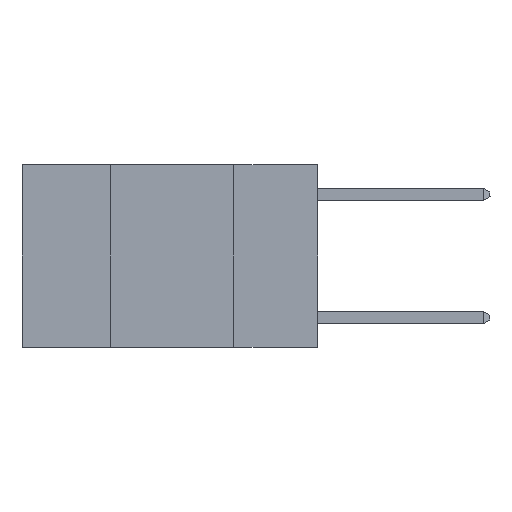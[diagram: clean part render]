
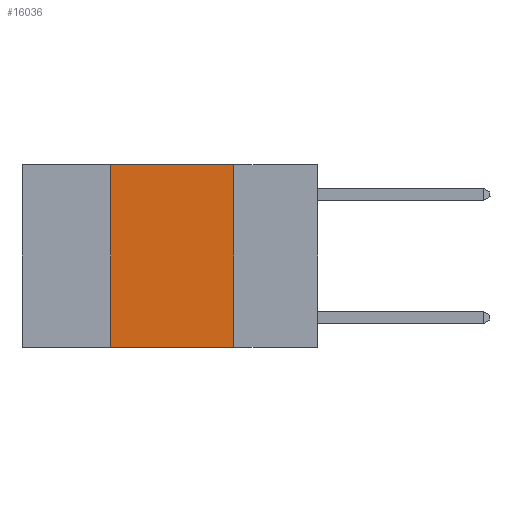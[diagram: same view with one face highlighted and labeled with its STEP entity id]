
A CAD part, left-side view. The second image highlights one B-rep face of the part: STEP entity #16036.
In plain terms, the highlighted planar face has unit normal (-1, 0, 0).
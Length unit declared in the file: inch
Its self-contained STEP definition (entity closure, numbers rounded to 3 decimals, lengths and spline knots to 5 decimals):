
#770 = CARTESIAN_POINT ( 'NONE',  ( 0., 0.42, 0. ) ) ;
#827 = VECTOR ( 'NONE', #1540, 39.37008 ) ;
#918 = LINE ( 'NONE', #11478, #5633 ) ;
#1540 = DIRECTION ( 'NONE',  ( 0., -1., 0. ) ) ;
#2212 = DIRECTION ( 'NONE',  ( 1., 0., 0. ) ) ;
#2724 = CARTESIAN_POINT ( 'NONE',  ( 0., 0.17, -0.37 ) ) ;
#3726 = EDGE_CURVE ( 'NONE', #4043, #10433, #17249, .T. ) ;
#4043 = VERTEX_POINT ( 'NONE', #13891 ) ;
#4356 = DIRECTION ( 'NONE',  ( 0., 0., -1. ) ) ;
#4636 = VECTOR ( 'NONE', #4356, 39.37008 ) ;
#5186 = AXIS2_PLACEMENT_3D ( 'NONE', #9815, #2212, #9720 ) ;
#5633 = VECTOR ( 'NONE', #13064, 39.37008 ) ;
#5973 = CARTESIAN_POINT ( 'NONE',  ( 0., 0.42, 0. ) ) ;
#7936 = FACE_OUTER_BOUND ( 'NONE', #10590, .T. ) ;
#8312 = CARTESIAN_POINT ( 'NONE',  ( 0., 0.17, 0. ) ) ;
#8603 = VERTEX_POINT ( 'NONE', #2724 ) ;
#8655 = EDGE_CURVE ( 'NONE', #10433, #9230, #13683, .T. ) ;
#9230 = VERTEX_POINT ( 'NONE', #13471 ) ;
#9720 = DIRECTION ( 'NONE',  ( 0., 0., -1. ) ) ;
#9815 = CARTESIAN_POINT ( 'NONE',  ( 0., 0.6, 0. ) ) ;
#10433 = VERTEX_POINT ( 'NONE', #5973 ) ;
#10590 = EDGE_LOOP ( 'NONE', ( #13961, #13755, #19386, #16271 ) ) ;
#10814 = CARTESIAN_POINT ( 'NONE',  ( 0., 0.6, 0. ) ) ;
#11478 = CARTESIAN_POINT ( 'NONE',  ( 0., 0.6, -0.37 ) ) ;
#11934 = EDGE_CURVE ( 'NONE', #4043, #8603, #918, .T. ) ;
#12489 = PLANE ( 'NONE',  #5186 ) ;
#13064 = DIRECTION ( 'NONE',  ( 0., -1., 0. ) ) ;
#13194 = EDGE_CURVE ( 'NONE', #9230, #8603, #15726, .T. ) ;
#13471 = CARTESIAN_POINT ( 'NONE',  ( 0., 0.17, 0. ) ) ;
#13683 = LINE ( 'NONE', #10814, #827 ) ;
#13755 = ORIENTED_EDGE ( 'NONE', *, *, #8655, .F. ) ;
#13891 = CARTESIAN_POINT ( 'NONE',  ( 0., 0.42, -0.37 ) ) ;
#13961 = ORIENTED_EDGE ( 'NONE', *, *, #13194, .F. ) ;
#15726 = LINE ( 'NONE', #8312, #4636 ) ;
#16036 = ADVANCED_FACE ( 'NONE', ( #7936 ), #12489, .F. ) ;
#16271 = ORIENTED_EDGE ( 'NONE', *, *, #11934, .T. ) ;
#17249 = LINE ( 'NONE', #770, #18064 ) ;
#17535 = DIRECTION ( 'NONE',  ( 0., 0., 1. ) ) ;
#18064 = VECTOR ( 'NONE', #17535, 39.37008 ) ;
#19386 = ORIENTED_EDGE ( 'NONE', *, *, #3726, .F. ) ;
